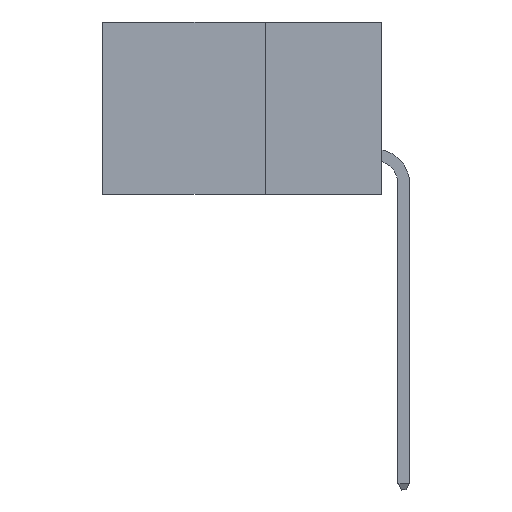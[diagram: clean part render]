
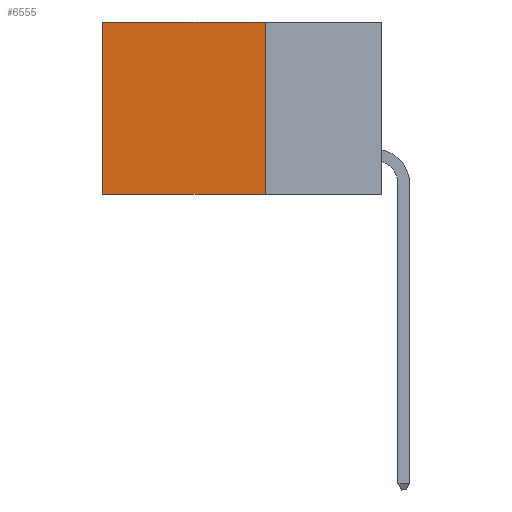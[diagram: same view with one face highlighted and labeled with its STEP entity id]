
A CAD part, left-side view. The second image highlights one B-rep face of the part: STEP entity #6555.
In plain terms, the highlighted planar face has unit normal (-1, 0, 0).
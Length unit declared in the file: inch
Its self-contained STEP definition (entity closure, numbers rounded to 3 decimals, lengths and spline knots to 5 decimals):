
#375 = CARTESIAN_POINT ( 'NONE',  ( 0.2875, 0.25, 0. ) ) ;
#394 = CARTESIAN_POINT ( 'NONE',  ( 0.2875, 0.25, -0.37 ) ) ;
#3366 = DIRECTION ( 'NONE',  ( 0., 0., -1. ) ) ;
#5412 = AXIS2_PLACEMENT_3D ( 'NONE', #37991, #13448, #38246 ) ;
#5974 = CARTESIAN_POINT ( 'NONE',  ( 0.2875, 0.25, -0.37 ) ) ;
#6448 = VERTEX_POINT ( 'NONE', #18342 ) ;
#6555 = ADVANCED_FACE ( 'NONE', ( #19522 ), #28578, .F. ) ;
#6574 = DIRECTION ( 'NONE',  ( 0., 1., 0. ) ) ;
#7398 = VECTOR ( 'NONE', #31617, 39.37008 ) ;
#7633 = DIRECTION ( 'NONE',  ( 0., 1., 0. ) ) ;
#7918 = LINE ( 'NONE', #34099, #7398 ) ;
#10178 = ORIENTED_EDGE ( 'NONE', *, *, #23764, .F. ) ;
#11289 = VECTOR ( 'NONE', #7633, 39.37008 ) ;
#13251 = LINE ( 'NONE', #394, #11289 ) ;
#13378 = EDGE_CURVE ( 'NONE', #23473, #36972, #7918, .T. ) ;
#13448 = DIRECTION ( 'NONE',  ( 1., 0., 0. ) ) ;
#15907 = VERTEX_POINT ( 'NONE', #5974 ) ;
#16248 = EDGE_CURVE ( 'NONE', #6448, #15907, #24185, .T. ) ;
#17308 = CARTESIAN_POINT ( 'NONE',  ( 0.2875, 0.6, -0.37 ) ) ;
#18342 = CARTESIAN_POINT ( 'NONE',  ( 0.2875, 0.25, 0. ) ) ;
#19522 = FACE_OUTER_BOUND ( 'NONE', #31435, .T. ) ;
#21723 = CARTESIAN_POINT ( 'NONE',  ( 0.2875, 0.6, 0. ) ) ;
#23473 = VERTEX_POINT ( 'NONE', #21723 ) ;
#23764 = EDGE_CURVE ( 'NONE', #15907, #36972, #13251, .T. ) ;
#24185 = LINE ( 'NONE', #375, #28066 ) ;
#24501 = CARTESIAN_POINT ( 'NONE',  ( 0.2875, 0.25, 0. ) ) ;
#25892 = EDGE_CURVE ( 'NONE', #6448, #23473, #34742, .T. ) ;
#28066 = VECTOR ( 'NONE', #3366, 39.37008 ) ;
#28578 = PLANE ( 'NONE',  #5412 ) ;
#30726 = ORIENTED_EDGE ( 'NONE', *, *, #16248, .F. ) ;
#31435 = EDGE_LOOP ( 'NONE', ( #33344, #10178, #30726, #38827 ) ) ;
#31617 = DIRECTION ( 'NONE',  ( 0., 0., -1. ) ) ;
#33344 = ORIENTED_EDGE ( 'NONE', *, *, #13378, .T. ) ;
#34099 = CARTESIAN_POINT ( 'NONE',  ( 0.2875, 0.6, 0. ) ) ;
#34742 = LINE ( 'NONE', #24501, #36723 ) ;
#36723 = VECTOR ( 'NONE', #6574, 39.37008 ) ;
#36972 = VERTEX_POINT ( 'NONE', #17308 ) ;
#37991 = CARTESIAN_POINT ( 'NONE',  ( 0.2875, 0.25, 0. ) ) ;
#38246 = DIRECTION ( 'NONE',  ( 0., 0., -1. ) ) ;
#38827 = ORIENTED_EDGE ( 'NONE', *, *, #25892, .T. ) ;
